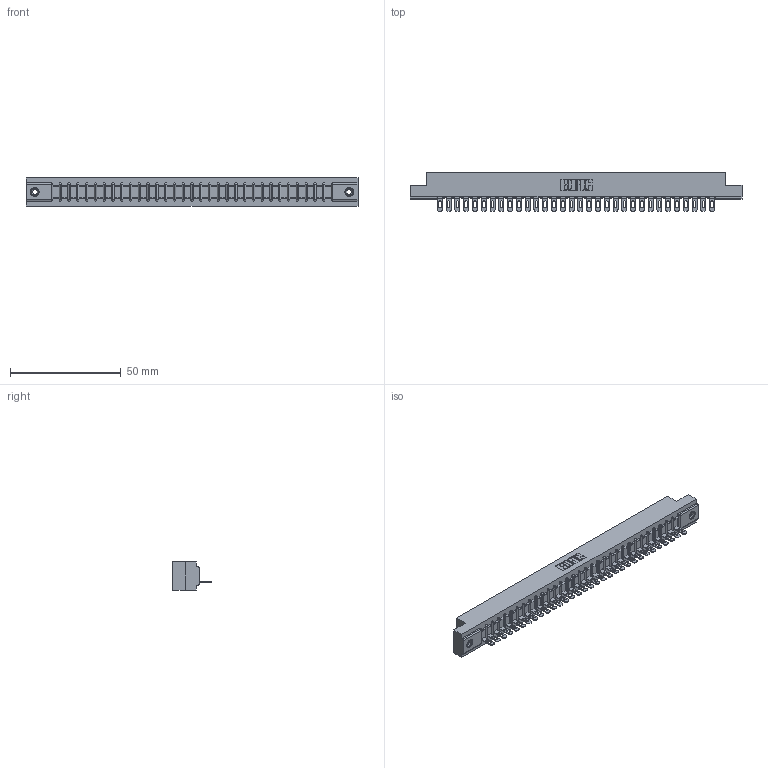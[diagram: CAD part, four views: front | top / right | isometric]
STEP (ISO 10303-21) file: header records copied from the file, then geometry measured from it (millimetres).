
FILE_DESCRIPTION (( 'STEP AP203' ), '1' );
FILE_NAME ('307-032-501-108.STEP', '2018-08-04T21:48:48', ( '' ), ( '' ), 'SwSTEP 2.0', 'SolidWorks 2016', '' );
FILE_SCHEMA (( 'CONFIG_CONTROL_DESIGN' ));
Length unit declared in the file: inch
Products named in the file (4): 345-250-001_345-250-003-102; 307-032-501-108; 307 Part_.156 Dia Mounting Holes; 307-290-002_501
Assembly tree (35 placements, depth 2):
  307-032-501-108
    307 Part_.156 Dia Mounting Holes
    307-290-002_501  x32
    345-250-001_345-250-003-102  x2
Bounding box: 149.81 x 17.42 x 12.7 mm (x, y, z)
Volume: 15978.3 mm3; surface area: 20107.3 mm2
Topology: 35 solids, 35 shells, 2643 faces, 8075 edges, 5286 vertices
Faces by surface type: plane 1510, cylinder 1051, sphere 66, cone 12, torus 4
Entity records: 30645 total; most frequent: CARTESIAN_POINT 5147, ORIENTED_EDGE 5130, DIRECTION 5019, EDGE_CURVE 2565, VECTOR 1955, LINE 1955, VERTEX_POINT 1660, AXIS2_PLACEMENT_3D 1532
